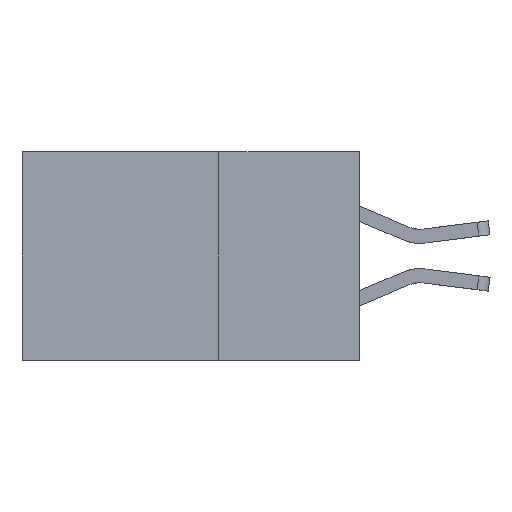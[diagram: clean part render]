
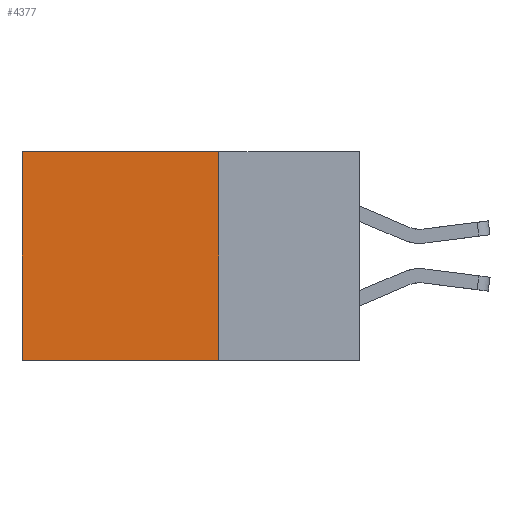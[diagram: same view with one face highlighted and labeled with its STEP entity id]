
A CAD part, left-side view. The second image highlights one B-rep face of the part: STEP entity #4377.
In plain terms, the highlighted planar face has unit normal (-1, 0, 0).
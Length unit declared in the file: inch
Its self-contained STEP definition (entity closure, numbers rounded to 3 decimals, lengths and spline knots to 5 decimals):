
#721 = PLANE ( 'NONE',  #9072 ) ;
#874 = ORIENTED_EDGE ( 'NONE', *, *, #4874, .T. ) ;
#883 = DIRECTION ( 'NONE',  ( 0., 0., -1. ) ) ;
#1195 = DIRECTION ( 'NONE',  ( 0., 0., -1. ) ) ;
#2260 = CARTESIAN_POINT ( 'NONE',  ( 0.2875, 0.6, -0.37 ) ) ;
#2342 = ORIENTED_EDGE ( 'NONE', *, *, #10800, .T. ) ;
#2950 = ORIENTED_EDGE ( 'NONE', *, *, #5859, .F. ) ;
#3104 = DIRECTION ( 'NONE',  ( 0., 1., 0. ) ) ;
#3201 = VERTEX_POINT ( 'NONE', #6524 ) ;
#3215 = VERTEX_POINT ( 'NONE', #12345 ) ;
#3358 = VECTOR ( 'NONE', #10177, 39.37008 ) ;
#3392 = CARTESIAN_POINT ( 'NONE',  ( 0.2875, 0.25, 0. ) ) ;
#3981 = ORIENTED_EDGE ( 'NONE', *, *, #8855, .F. ) ;
#4143 = DIRECTION ( 'NONE',  ( 0., 0., -1. ) ) ;
#4377 = ADVANCED_FACE ( 'NONE', ( #12491 ), #721, .F. ) ;
#4599 = EDGE_LOOP ( 'NONE', ( #874, #2950, #3981, #2342 ) ) ;
#4874 = EDGE_CURVE ( 'NONE', #3201, #9462, #12343, .T. ) ;
#4952 = LINE ( 'NONE', #8910, #7360 ) ;
#5030 = CARTESIAN_POINT ( 'NONE',  ( 0.2875, 0.25, 0. ) ) ;
#5859 = EDGE_CURVE ( 'NONE', #3215, #9462, #4952, .T. ) ;
#6524 = CARTESIAN_POINT ( 'NONE',  ( 0.2875, 0.6, 0. ) ) ;
#6682 = VECTOR ( 'NONE', #4143, 39.37008 ) ;
#7360 = VECTOR ( 'NONE', #3104, 39.37008 ) ;
#7597 = DIRECTION ( 'NONE',  ( 1., 0., 0. ) ) ;
#7928 = CARTESIAN_POINT ( 'NONE',  ( 0.2875, 0.6, 0. ) ) ;
#8040 = VERTEX_POINT ( 'NONE', #11101 ) ;
#8855 = EDGE_CURVE ( 'NONE', #8040, #3215, #11637, .T. ) ;
#8910 = CARTESIAN_POINT ( 'NONE',  ( 0.2875, 0.25, -0.37 ) ) ;
#9072 = AXIS2_PLACEMENT_3D ( 'NONE', #12443, #7597, #883 ) ;
#9462 = VERTEX_POINT ( 'NONE', #2260 ) ;
#10177 = DIRECTION ( 'NONE',  ( 0., 1., 0. ) ) ;
#10800 = EDGE_CURVE ( 'NONE', #8040, #3201, #11761, .T. ) ;
#11101 = CARTESIAN_POINT ( 'NONE',  ( 0.2875, 0.25, 0. ) ) ;
#11291 = VECTOR ( 'NONE', #1195, 39.37008 ) ;
#11637 = LINE ( 'NONE', #5030, #6682 ) ;
#11761 = LINE ( 'NONE', #3392, #3358 ) ;
#12343 = LINE ( 'NONE', #7928, #11291 ) ;
#12345 = CARTESIAN_POINT ( 'NONE',  ( 0.2875, 0.25, -0.37 ) ) ;
#12443 = CARTESIAN_POINT ( 'NONE',  ( 0.2875, 0.25, 0. ) ) ;
#12491 = FACE_OUTER_BOUND ( 'NONE', #4599, .T. ) ;
